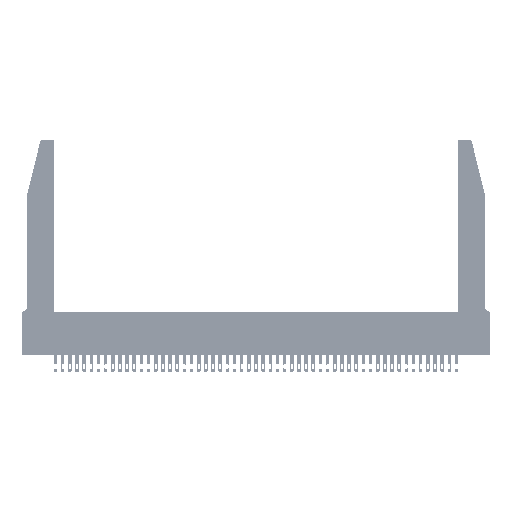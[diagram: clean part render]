
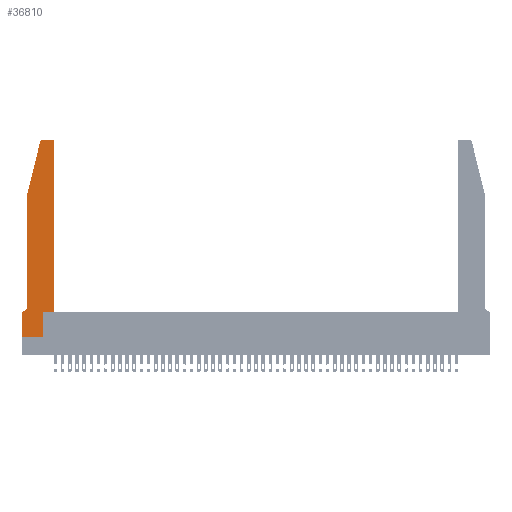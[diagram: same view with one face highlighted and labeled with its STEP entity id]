
A CAD part, top view. The second image highlights one B-rep face of the part: STEP entity #36810.
In plain terms, the highlighted planar face has unit normal (0, 0, 1).
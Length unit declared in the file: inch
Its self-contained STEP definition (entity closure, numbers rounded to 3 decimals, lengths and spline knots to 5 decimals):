
#679 = EDGE_CURVE ( 'NONE', #37850, #5278, #12460, .T. ) ;
#1607 = VECTOR ( 'NONE', #29509, 39.37008 ) ;
#1949 = VERTEX_POINT ( 'NONE', #7021 ) ;
#2398 = CARTESIAN_POINT ( 'NONE',  ( 0.4205, 2.75, 0.37 ) ) ;
#2401 = CARTESIAN_POINT ( 'NONE',  ( 0.2865, 0., 0.37 ) ) ;
#2661 = AXIS2_PLACEMENT_3D ( 'NONE', #41733, #27342, #9105 ) ;
#2875 = DIRECTION ( 'NONE',  ( 0., -1., 0. ) ) ;
#3086 = ORIENTED_EDGE ( 'NONE', *, *, #7858, .T. ) ;
#3092 = PLANE ( 'NONE',  #19995 ) ;
#3449 = DIRECTION ( 'NONE',  ( 0., 0., 1. ) ) ;
#3597 = DIRECTION ( 'NONE',  ( 1., 0., 0. ) ) ;
#4036 = CARTESIAN_POINT ( 'NONE',  ( 0.284, 2.72, 0.37 ) ) ;
#4737 = EDGE_CURVE ( 'NONE', #38519, #42172, #26996, .T. ) ;
#4878 = CARTESIAN_POINT ( 'NONE',  ( 0.4505, 0.35, 0.37 ) ) ;
#4993 = LINE ( 'NONE', #47154, #8991 ) ;
#5103 = ORIENTED_EDGE ( 'NONE', *, *, #34095, .T. ) ;
#5278 = VERTEX_POINT ( 'NONE', #2401 ) ;
#5681 = CARTESIAN_POINT ( 'NONE',  ( 0.0755, 2., 0.37 ) ) ;
#6526 = ORIENTED_EDGE ( 'NONE', *, *, #4737, .T. ) ;
#7021 = CARTESIAN_POINT ( 'NONE',  ( 0.0755, 2., 0.37 ) ) ;
#7858 = EDGE_CURVE ( 'NONE', #16032, #38519, #23848, .T. ) ;
#8302 = CARTESIAN_POINT ( 'NONE',  ( 0.0055, 0.35, 0.37 ) ) ;
#8991 = VECTOR ( 'NONE', #33660, 39.37008 ) ;
#9105 = DIRECTION ( 'NONE',  ( 1., 0., 0. ) ) ;
#10931 = DIRECTION ( 'NONE',  ( 1., 0., 0. ) ) ;
#12034 = CARTESIAN_POINT ( 'NONE',  ( 0., 0.35, 0.37 ) ) ;
#12460 = LINE ( 'NONE', #13714, #41673 ) ;
#13018 = DIRECTION ( 'NONE',  ( -0.239, -0.971, 0. ) ) ;
#13427 = LINE ( 'NONE', #29473, #30563 ) ;
#13714 = CARTESIAN_POINT ( 'NONE',  ( 0., 0., 0.37 ) ) ;
#16032 = VERTEX_POINT ( 'NONE', #18974 ) ;
#16309 = VECTOR ( 'NONE', #2875, 39.37008 ) ;
#18606 = VECTOR ( 'NONE', #13018, 39.37008 ) ;
#18674 = EDGE_CURVE ( 'NONE', #5278, #43950, #25674, .T. ) ;
#18974 = CARTESIAN_POINT ( 'NONE',  ( 0.4505, 2.72, 0.37 ) ) ;
#19138 = CARTESIAN_POINT ( 'NONE',  ( 0.0755, 0.42, 0.37 ) ) ;
#19956 = LINE ( 'NONE', #4878, #1607 ) ;
#19995 = AXIS2_PLACEMENT_3D ( 'NONE', #32510, #32351, #36365 ) ;
#20489 = DIRECTION ( 'NONE',  ( 0., 1., 0. ) ) ;
#20590 = CARTESIAN_POINT ( 'NONE',  ( 0., 0., 0.37 ) ) ;
#21139 = DIRECTION ( 'NONE',  ( -1., 0., 0. ) ) ;
#21721 = VECTOR ( 'NONE', #20489, 39.37008 ) ;
#22571 = EDGE_CURVE ( 'NONE', #43950, #35691, #4993, .T. ) ;
#23352 = AXIS2_PLACEMENT_3D ( 'NONE', #4036, #3449, #10931 ) ;
#23721 = CARTESIAN_POINT ( 'NONE',  ( 0.25487, 2.72718, 0.37 ) ) ;
#23848 = CIRCLE ( 'NONE', #2661, 0.03 ) ;
#23883 = VERTEX_POINT ( 'NONE', #8302 ) ;
#24757 = CARTESIAN_POINT ( 'NONE',  ( 0., 0., 0.37 ) ) ;
#24869 = DIRECTION ( 'NONE',  ( -1., 0., 0. ) ) ;
#25563 = FACE_OUTER_BOUND ( 'NONE', #41353, .T. ) ;
#25634 = ORIENTED_EDGE ( 'NONE', *, *, #18674, .T. ) ;
#25674 = LINE ( 'NONE', #42556, #21721 ) ;
#26295 = ORIENTED_EDGE ( 'NONE', *, *, #40228, .T. ) ;
#26395 = VERTEX_POINT ( 'NONE', #19138 ) ;
#26540 = LINE ( 'NONE', #24757, #16309 ) ;
#26996 = LINE ( 'NONE', #28426, #29318 ) ;
#27045 = DIRECTION ( 'NONE',  ( 0., -1., 0. ) ) ;
#27342 = DIRECTION ( 'NONE',  ( 0., 0., 1. ) ) ;
#28246 = ORIENTED_EDGE ( 'NONE', *, *, #22571, .T. ) ;
#28426 = CARTESIAN_POINT ( 'NONE',  ( 0.2605, 2.75, 0.37 ) ) ;
#29318 = VECTOR ( 'NONE', #24869, 39.37008 ) ;
#29473 = CARTESIAN_POINT ( 'NONE',  ( 0.0755, 2., 0.37 ) ) ;
#29509 = DIRECTION ( 'NONE',  ( 0., 1., 0. ) ) ;
#30156 = ORIENTED_EDGE ( 'NONE', *, *, #41903, .T. ) ;
#30286 = CIRCLE ( 'NONE', #32578, 0.07 ) ;
#30563 = VECTOR ( 'NONE', #27045, 39.37008 ) ;
#31856 = LINE ( 'NONE', #5681, #18606 ) ;
#31930 = DIRECTION ( 'NONE',  ( -1., 0., 0. ) ) ;
#32351 = DIRECTION ( 'NONE',  ( 0., 0., 1. ) ) ;
#32383 = CARTESIAN_POINT ( 'NONE',  ( 0.284, 2.75, 0.37 ) ) ;
#32510 = CARTESIAN_POINT ( 'NONE',  ( 0., 0.35, 0.37 ) ) ;
#32578 = AXIS2_PLACEMENT_3D ( 'NONE', #35948, #43093, #31930 ) ;
#32754 = LINE ( 'NONE', #43533, #45328 ) ;
#33660 = DIRECTION ( 'NONE',  ( 1., 0., 0. ) ) ;
#34095 = EDGE_CURVE ( 'NONE', #23883, #44794, #32754, .T. ) ;
#34194 = ORIENTED_EDGE ( 'NONE', *, *, #43297, .T. ) ;
#34196 = CIRCLE ( 'NONE', #23352, 0.03 ) ;
#35193 = VERTEX_POINT ( 'NONE', #23721 ) ;
#35284 = EDGE_CURVE ( 'NONE', #26395, #23883, #30286, .T. ) ;
#35691 = VERTEX_POINT ( 'NONE', #44252 ) ;
#35906 = ORIENTED_EDGE ( 'NONE', *, *, #679, .T. ) ;
#35948 = CARTESIAN_POINT ( 'NONE',  ( 0.0055, 0.42, 0.37 ) ) ;
#36365 = DIRECTION ( 'NONE',  ( 1., 0., 0. ) ) ;
#36372 = EDGE_CURVE ( 'NONE', #42172, #35193, #34196, .T. ) ;
#36810 = ADVANCED_FACE ( 'NONE', ( #25563 ), #3092, .T. ) ;
#37850 = VERTEX_POINT ( 'NONE', #20590 ) ;
#38519 = VERTEX_POINT ( 'NONE', #2398 ) ;
#38945 = EDGE_CURVE ( 'NONE', #1949, #26395, #13427, .T. ) ;
#40228 = EDGE_CURVE ( 'NONE', #35691, #16032, #19956, .T. ) ;
#41353 = EDGE_LOOP ( 'NONE', ( #6526, #44438, #30156, #46256, #42609, #5103, #34194, #35906, #25634, #28246, #26295, #3086 ) ) ;
#41673 = VECTOR ( 'NONE', #3597, 39.37008 ) ;
#41733 = CARTESIAN_POINT ( 'NONE',  ( 0.4205, 2.72, 0.37 ) ) ;
#41903 = EDGE_CURVE ( 'NONE', #35193, #1949, #31856, .T. ) ;
#42172 = VERTEX_POINT ( 'NONE', #32383 ) ;
#42556 = CARTESIAN_POINT ( 'NONE',  ( 0.2865, 0.35, 0.37 ) ) ;
#42609 = ORIENTED_EDGE ( 'NONE', *, *, #35284, .T. ) ;
#42961 = CARTESIAN_POINT ( 'NONE',  ( 0.2865, 0.35, 0.37 ) ) ;
#43093 = DIRECTION ( 'NONE',  ( 0., 0., -1. ) ) ;
#43297 = EDGE_CURVE ( 'NONE', #44794, #37850, #26540, .T. ) ;
#43533 = CARTESIAN_POINT ( 'NONE',  ( 0.0755, 0.35, 0.37 ) ) ;
#43950 = VERTEX_POINT ( 'NONE', #42961 ) ;
#44252 = CARTESIAN_POINT ( 'NONE',  ( 0.4505, 0.35, 0.37 ) ) ;
#44438 = ORIENTED_EDGE ( 'NONE', *, *, #36372, .T. ) ;
#44794 = VERTEX_POINT ( 'NONE', #12034 ) ;
#45328 = VECTOR ( 'NONE', #21139, 39.37008 ) ;
#46256 = ORIENTED_EDGE ( 'NONE', *, *, #38945, .T. ) ;
#47154 = CARTESIAN_POINT ( 'NONE',  ( 0.4505, 0.35, 0.37 ) ) ;
